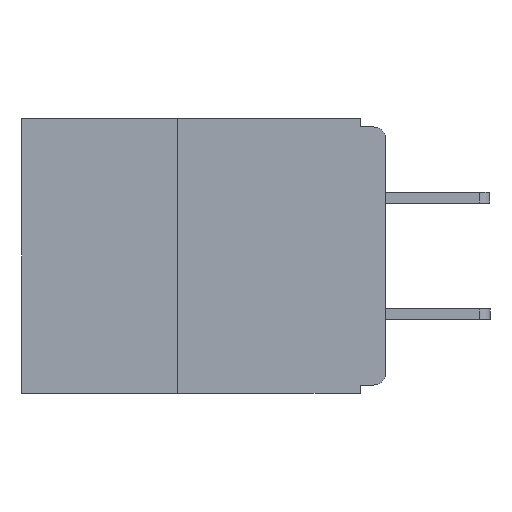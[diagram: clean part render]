
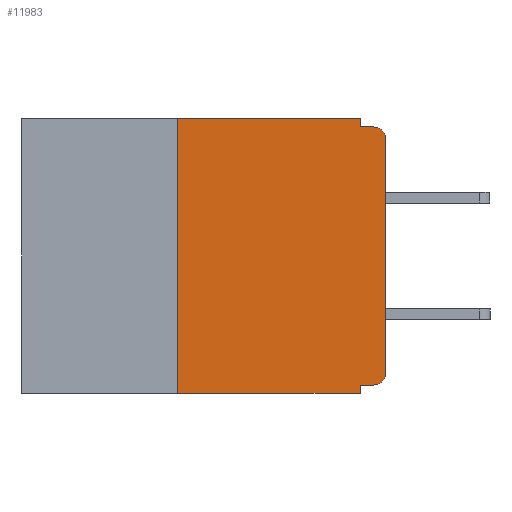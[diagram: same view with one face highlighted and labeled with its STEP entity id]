
A CAD part, left-side view. The second image highlights one B-rep face of the part: STEP entity #11983.
In plain terms, the highlighted planar face has unit normal (-1, 0, 0).
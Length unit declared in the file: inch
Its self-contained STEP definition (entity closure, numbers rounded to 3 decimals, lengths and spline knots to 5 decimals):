
#172 = VERTEX_POINT ( 'NONE', #17657 ) ;
#226 = DIRECTION ( 'NONE',  ( -1., 0., 0. ) ) ;
#348 = VERTEX_POINT ( 'NONE', #9170 ) ;
#533 = CARTESIAN_POINT ( 'NONE',  ( 0., 0.437, 0. ) ) ;
#1564 = VERTEX_POINT ( 'NONE', #27144 ) ;
#2698 = CARTESIAN_POINT ( 'NONE',  ( 0., 0.031, -0.33 ) ) ;
#2952 = CARTESIAN_POINT ( 'NONE',  ( 0., 0.25, -0.33 ) ) ;
#3982 = CARTESIAN_POINT ( 'NONE',  ( 0., 0., 0. ) ) ;
#4120 = VECTOR ( 'NONE', #15498, 39.37008 ) ;
#4269 = VERTEX_POINT ( 'NONE', #8655 ) ;
#4389 = LINE ( 'NONE', #2952, #22132 ) ;
#5187 = AXIS2_PLACEMENT_3D ( 'NONE', #13677, #226, #15960 ) ;
#6282 = DIRECTION ( 'NONE',  ( 0., 0., 1. ) ) ;
#6391 = VERTEX_POINT ( 'NONE', #9025 ) ;
#6843 = DIRECTION ( 'NONE',  ( 0., -1., 0. ) ) ;
#7334 = CARTESIAN_POINT ( 'NONE',  ( 0., 0.031, -0.33 ) ) ;
#7531 = EDGE_CURVE ( 'NONE', #4269, #348, #17804, .T. ) ;
#7758 = VERTEX_POINT ( 'NONE', #8825 ) ;
#8449 = EDGE_CURVE ( 'NONE', #1564, #172, #22142, .T. ) ;
#8655 = CARTESIAN_POINT ( 'NONE',  ( 0., 0.015, -0.32 ) ) ;
#8825 = CARTESIAN_POINT ( 'NONE',  ( 0., 0., -0.025 ) ) ;
#9025 = CARTESIAN_POINT ( 'NONE',  ( 0., 0.25, 0. ) ) ;
#9170 = CARTESIAN_POINT ( 'NONE',  ( 0., 0., -0.305 ) ) ;
#9583 = DIRECTION ( 'NONE',  ( 0., 0., -1. ) ) ;
#9589 = VECTOR ( 'NONE', #22162, 39.37008 ) ;
#9868 = CIRCLE ( 'NONE', #5187, 0.015 ) ;
#10304 = CARTESIAN_POINT ( 'NONE',  ( 0., 0.015, -0.305 ) ) ;
#10379 = AXIS2_PLACEMENT_3D ( 'NONE', #10304, #25709, #12519 ) ;
#10775 = AXIS2_PLACEMENT_3D ( 'NONE', #533, #22831, #9583 ) ;
#11731 = VECTOR ( 'NONE', #6843, 39.37008 ) ;
#11983 = ADVANCED_FACE ( 'NONE', ( #20961 ), #20662, .F. ) ;
#12519 = DIRECTION ( 'NONE',  ( 0., 0., -1. ) ) ;
#12655 = VERTEX_POINT ( 'NONE', #2698 ) ;
#13260 = EDGE_CURVE ( 'NONE', #17238, #12655, #19741, .T. ) ;
#13519 = LINE ( 'NONE', #3982, #24545 ) ;
#13677 = CARTESIAN_POINT ( 'NONE',  ( 0., 0.015, -0.025 ) ) ;
#14723 = DIRECTION ( 'NONE',  ( 0., -1., 0. ) ) ;
#15011 = EDGE_CURVE ( 'NONE', #7758, #172, #9868, .T. ) ;
#15353 = LINE ( 'NONE', #22096, #4120 ) ;
#15498 = DIRECTION ( 'NONE',  ( 0., -1., 0. ) ) ;
#15559 = LINE ( 'NONE', #24356, #9589 ) ;
#15960 = DIRECTION ( 'NONE',  ( 0., 0., -1. ) ) ;
#16130 = ORIENTED_EDGE ( 'NONE', *, *, #18965, .T. ) ;
#16131 = VERTEX_POINT ( 'NONE', #26790 ) ;
#16268 = ORIENTED_EDGE ( 'NONE', *, *, #15011, .T. ) ;
#16486 = ORIENTED_EDGE ( 'NONE', *, *, #8449, .F. ) ;
#16675 = ORIENTED_EDGE ( 'NONE', *, *, #22147, .F. ) ;
#17020 = ORIENTED_EDGE ( 'NONE', *, *, #21941, .F. ) ;
#17196 = ORIENTED_EDGE ( 'NONE', *, *, #19302, .F. ) ;
#17238 = VERTEX_POINT ( 'NONE', #17982 ) ;
#17265 = ORIENTED_EDGE ( 'NONE', *, *, #17801, .T. ) ;
#17489 = ORIENTED_EDGE ( 'NONE', *, *, #13260, .F. ) ;
#17621 = ORIENTED_EDGE ( 'NONE', *, *, #25278, .F. ) ;
#17657 = CARTESIAN_POINT ( 'NONE',  ( 0., 0.015, -0.01 ) ) ;
#17747 = CARTESIAN_POINT ( 'NONE',  ( 0., 0.031, 0. ) ) ;
#17801 = EDGE_CURVE ( 'NONE', #20602, #12655, #15353, .T. ) ;
#17804 = CIRCLE ( 'NONE', #10379, 0.015 ) ;
#17882 = ORIENTED_EDGE ( 'NONE', *, *, #7531, .T. ) ;
#17982 = CARTESIAN_POINT ( 'NONE',  ( 0., 0.031, -0.32 ) ) ;
#18692 = DIRECTION ( 'NONE',  ( 0., 0., 1. ) ) ;
#18965 = EDGE_CURVE ( 'NONE', #348, #7758, #13519, .T. ) ;
#19087 = VECTOR ( 'NONE', #27133, 39.37008 ) ;
#19208 = CARTESIAN_POINT ( 'NONE',  ( 0., 0.25, -0.33 ) ) ;
#19302 = EDGE_CURVE ( 'NONE', #20602, #6391, #4389, .T. ) ;
#19671 = VECTOR ( 'NONE', #14723, 39.37008 ) ;
#19741 = LINE ( 'NONE', #7334, #19087 ) ;
#20602 = VERTEX_POINT ( 'NONE', #19208 ) ;
#20649 = LINE ( 'NONE', #17747, #22000 ) ;
#20662 = PLANE ( 'NONE',  #10775 ) ;
#20961 = FACE_OUTER_BOUND ( 'NONE', #28573, .T. ) ;
#21259 = CARTESIAN_POINT ( 'NONE',  ( 0., 0.437, 0. ) ) ;
#21941 = EDGE_CURVE ( 'NONE', #6391, #16131, #25420, .T. ) ;
#22000 = VECTOR ( 'NONE', #22004, 39.37008 ) ;
#22004 = DIRECTION ( 'NONE',  ( 0., 0., -1. ) ) ;
#22096 = CARTESIAN_POINT ( 'NONE',  ( 0., 0.437, -0.33 ) ) ;
#22132 = VECTOR ( 'NONE', #18692, 39.37008 ) ;
#22142 = LINE ( 'NONE', #22238, #11731 ) ;
#22147 = EDGE_CURVE ( 'NONE', #16131, #1564, #20649, .T. ) ;
#22162 = DIRECTION ( 'NONE',  ( 0., 1., 0. ) ) ;
#22238 = CARTESIAN_POINT ( 'NONE',  ( 0., 0., -0.01 ) ) ;
#22831 = DIRECTION ( 'NONE',  ( 1., 0., 0. ) ) ;
#24356 = CARTESIAN_POINT ( 'NONE',  ( 0., 0., -0.32 ) ) ;
#24545 = VECTOR ( 'NONE', #6282, 39.37008 ) ;
#25278 = EDGE_CURVE ( 'NONE', #4269, #17238, #15559, .T. ) ;
#25420 = LINE ( 'NONE', #21259, #19671 ) ;
#25709 = DIRECTION ( 'NONE',  ( -1., 0., 0. ) ) ;
#26790 = CARTESIAN_POINT ( 'NONE',  ( 0., 0.031, 0. ) ) ;
#27133 = DIRECTION ( 'NONE',  ( 0., 0., -1. ) ) ;
#27144 = CARTESIAN_POINT ( 'NONE',  ( 0., 0.031, -0.01 ) ) ;
#28573 = EDGE_LOOP ( 'NONE', ( #16130, #16268, #16486, #16675, #17020, #17196, #17265, #17489, #17621, #17882 ) ) ;
